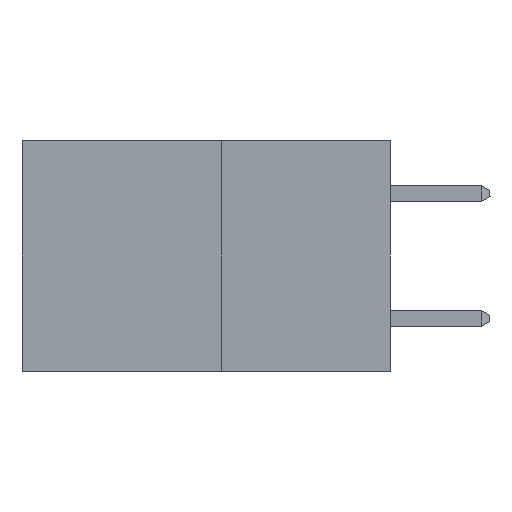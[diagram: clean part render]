
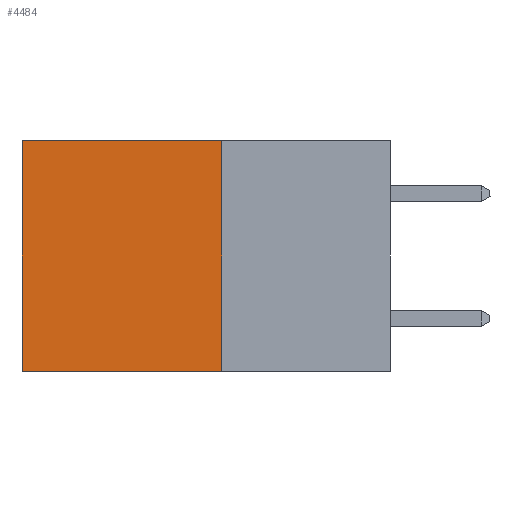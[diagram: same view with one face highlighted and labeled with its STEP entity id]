
A CAD part, left-side view. The second image highlights one B-rep face of the part: STEP entity #4484.
In plain terms, the highlighted planar face has unit normal (-1, 0, 0).
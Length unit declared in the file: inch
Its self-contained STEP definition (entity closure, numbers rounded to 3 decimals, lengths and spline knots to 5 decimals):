
#36 = CARTESIAN_POINT ( 'NONE',  ( 0.277, 0.27, 0. ) ) ;
#200 = FACE_OUTER_BOUND ( 'NONE', #5214, .T. ) ;
#294 = LINE ( 'NONE', #3094, #7039 ) ;
#428 = LINE ( 'NONE', #7979, #10685 ) ;
#884 = VERTEX_POINT ( 'NONE', #8584 ) ;
#1278 = DIRECTION ( 'NONE',  ( 1., 0., 0. ) ) ;
#1505 = VERTEX_POINT ( 'NONE', #9841 ) ;
#1685 = CARTESIAN_POINT ( 'NONE',  ( 0.277, 0.27, -0.37 ) ) ;
#1802 = AXIS2_PLACEMENT_3D ( 'NONE', #14719, #1278, #11024 ) ;
#2388 = ORIENTED_EDGE ( 'NONE', *, *, #3421, .T. ) ;
#3094 = CARTESIAN_POINT ( 'NONE',  ( 0.277, 0.27, -0.37 ) ) ;
#3201 = CARTESIAN_POINT ( 'NONE',  ( 0.277, 0.27, -0.37 ) ) ;
#3421 = EDGE_CURVE ( 'NONE', #12064, #884, #12672, .T. ) ;
#3966 = ORIENTED_EDGE ( 'NONE', *, *, #3982, .T. ) ;
#3982 = EDGE_CURVE ( 'NONE', #884, #1505, #428, .T. ) ;
#4460 = DIRECTION ( 'NONE',  ( 0., 0., -1. ) ) ;
#4484 = ADVANCED_FACE ( 'NONE', ( #200 ), #7885, .F. ) ;
#5214 = EDGE_LOOP ( 'NONE', ( #3966, #5756, #13060, #2388 ) ) ;
#5349 = DIRECTION ( 'NONE',  ( 0., 0., -1. ) ) ;
#5756 = ORIENTED_EDGE ( 'NONE', *, *, #13769, .F. ) ;
#7039 = VECTOR ( 'NONE', #4460, 39.37008 ) ;
#7161 = DIRECTION ( 'NONE',  ( 0., 1., 0. ) ) ;
#7359 = VERTEX_POINT ( 'NONE', #3201 ) ;
#7446 = LINE ( 'NONE', #1685, #13445 ) ;
#7885 = PLANE ( 'NONE',  #1802 ) ;
#7979 = CARTESIAN_POINT ( 'NONE',  ( 0.277, 0.59, -0.37 ) ) ;
#8584 = CARTESIAN_POINT ( 'NONE',  ( 0.277, 0.59, 0. ) ) ;
#9841 = CARTESIAN_POINT ( 'NONE',  ( 0.277, 0.59, -0.37 ) ) ;
#10611 = CARTESIAN_POINT ( 'NONE',  ( 0.277, 0.27, 0. ) ) ;
#10685 = VECTOR ( 'NONE', #5349, 39.37008 ) ;
#10725 = DIRECTION ( 'NONE',  ( 0., 1., 0. ) ) ;
#11024 = DIRECTION ( 'NONE',  ( 0., 0., -1. ) ) ;
#12064 = VERTEX_POINT ( 'NONE', #36 ) ;
#12672 = LINE ( 'NONE', #10611, #15083 ) ;
#13060 = ORIENTED_EDGE ( 'NONE', *, *, #13760, .F. ) ;
#13445 = VECTOR ( 'NONE', #7161, 39.37008 ) ;
#13760 = EDGE_CURVE ( 'NONE', #12064, #7359, #294, .T. ) ;
#13769 = EDGE_CURVE ( 'NONE', #7359, #1505, #7446, .T. ) ;
#14719 = CARTESIAN_POINT ( 'NONE',  ( 0.277, 0.27, -0.37 ) ) ;
#15083 = VECTOR ( 'NONE', #10725, 39.37008 ) ;
